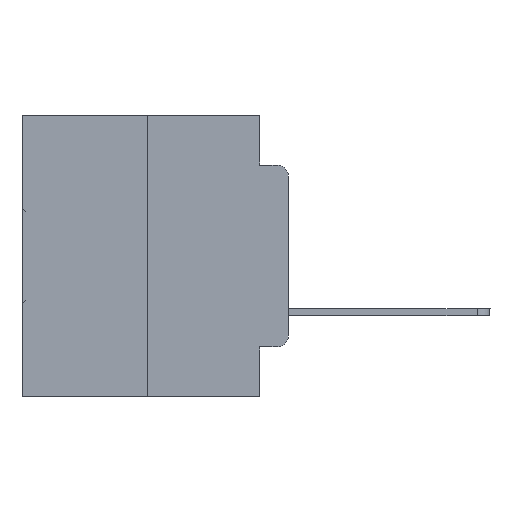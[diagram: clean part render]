
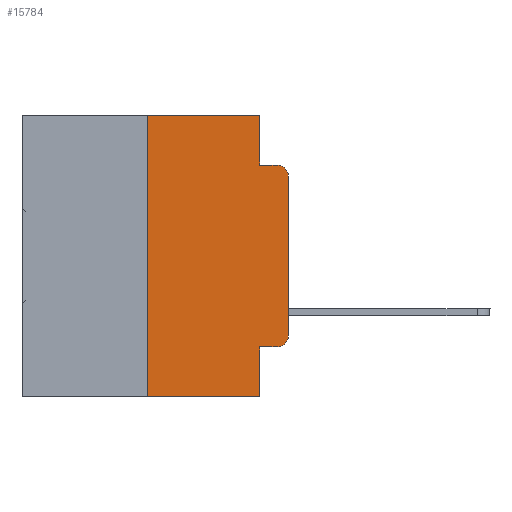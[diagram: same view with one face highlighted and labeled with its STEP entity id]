
A CAD part, left-side view. The second image highlights one B-rep face of the part: STEP entity #15784.
In plain terms, the highlighted planar face has unit normal (-1, 0, 0).
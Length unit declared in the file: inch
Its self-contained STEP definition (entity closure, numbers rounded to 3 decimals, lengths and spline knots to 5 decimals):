
#162 = VERTEX_POINT ( 'NONE', #5571 ) ;
#623 = LINE ( 'NONE', #5363, #6239 ) ;
#1288 = VERTEX_POINT ( 'NONE', #12887 ) ;
#1363 = AXIS2_PLACEMENT_3D ( 'NONE', #4456, #24964, #9524 ) ;
#1486 = VECTOR ( 'NONE', #15896, 39.37008 ) ;
#2655 = VERTEX_POINT ( 'NONE', #20567 ) ;
#3186 = CARTESIAN_POINT ( 'NONE',  ( 0., 0.051, 0. ) ) ;
#3588 = CIRCLE ( 'NONE', #24686, 0.02 ) ;
#3691 = VERTEX_POINT ( 'NONE', #13807 ) ;
#4365 = ORIENTED_EDGE ( 'NONE', *, *, #14681, .F. ) ;
#4456 = CARTESIAN_POINT ( 'NONE',  ( 0., 0.02, -0.3915 ) ) ;
#4658 = VECTOR ( 'NONE', #15212, 39.37008 ) ;
#4673 = CARTESIAN_POINT ( 'NONE',  ( 0., 0.051, -0.0885 ) ) ;
#4717 = VERTEX_POINT ( 'NONE', #15703 ) ;
#4820 = VECTOR ( 'NONE', #15538, 39.37008 ) ;
#4888 = EDGE_LOOP ( 'NONE', ( #22694, #17492, #4365, #20376, #17443, #29692, #32384, #18945, #14349, #13107 ) ) ;
#5183 = LINE ( 'NONE', #20302, #4820 ) ;
#5363 = CARTESIAN_POINT ( 'NONE',  ( 0., 0.051, -0.0885 ) ) ;
#5571 = CARTESIAN_POINT ( 'NONE',  ( 0., 0., -0.1085 ) ) ;
#6239 = VECTOR ( 'NONE', #21307, 39.37008 ) ;
#6391 = EDGE_CURVE ( 'NONE', #1288, #162, #12624, .T. ) ;
#7140 = DIRECTION ( 'NONE',  ( 1., 0., 0. ) ) ;
#7527 = DIRECTION ( 'NONE',  ( 0., 0., -1. ) ) ;
#7736 = CARTESIAN_POINT ( 'NONE',  ( 0., 0.473, 0. ) ) ;
#8259 = CARTESIAN_POINT ( 'NONE',  ( 0., 0.051, -0.4115 ) ) ;
#8658 = VECTOR ( 'NONE', #22796, 39.37008 ) ;
#9189 = VERTEX_POINT ( 'NONE', #19619 ) ;
#9524 = DIRECTION ( 'NONE',  ( 0., 0., -1. ) ) ;
#12209 = FACE_OUTER_BOUND ( 'NONE', #4888, .T. ) ;
#12624 = LINE ( 'NONE', #31084, #8658 ) ;
#12654 = CARTESIAN_POINT ( 'NONE',  ( 0., 0.051, 0. ) ) ;
#12887 = CARTESIAN_POINT ( 'NONE',  ( 0., 0., -0.3915 ) ) ;
#12994 = EDGE_CURVE ( 'NONE', #30410, #27808, #28955, .T. ) ;
#13107 = ORIENTED_EDGE ( 'NONE', *, *, #15301, .T. ) ;
#13537 = DIRECTION ( 'NONE',  ( 0., 0., -1. ) ) ;
#13544 = CARTESIAN_POINT ( 'NONE',  ( 0., 0.02, -0.4115 ) ) ;
#13807 = CARTESIAN_POINT ( 'NONE',  ( 0., 0.051, -0.4115 ) ) ;
#14231 = VERTEX_POINT ( 'NONE', #13544 ) ;
#14349 = ORIENTED_EDGE ( 'NONE', *, *, #17168, .T. ) ;
#14492 = DIRECTION ( 'NONE',  ( 0., -1., 0. ) ) ;
#14582 = CARTESIAN_POINT ( 'NONE',  ( 0., 0.051, 0. ) ) ;
#14681 = EDGE_CURVE ( 'NONE', #27808, #23661, #623, .T. ) ;
#15212 = DIRECTION ( 'NONE',  ( 0., 0., -1. ) ) ;
#15301 = EDGE_CURVE ( 'NONE', #14231, #1288, #31148, .T. ) ;
#15538 = DIRECTION ( 'NONE',  ( 0., 0., 1. ) ) ;
#15703 = CARTESIAN_POINT ( 'NONE',  ( 0., 0.25, 0. ) ) ;
#15784 = ADVANCED_FACE ( 'NONE', ( #12209 ), #22550, .F. ) ;
#15896 = DIRECTION ( 'NONE',  ( 0., -1., 0. ) ) ;
#17168 = EDGE_CURVE ( 'NONE', #3691, #14231, #26563, .T. ) ;
#17443 = ORIENTED_EDGE ( 'NONE', *, *, #21016, .F. ) ;
#17492 = ORIENTED_EDGE ( 'NONE', *, *, #29667, .T. ) ;
#17595 = CARTESIAN_POINT ( 'NONE',  ( 0., 0.02, -0.0885 ) ) ;
#18201 = VECTOR ( 'NONE', #13537, 39.37008 ) ;
#18945 = ORIENTED_EDGE ( 'NONE', *, *, #29339, .F. ) ;
#19619 = CARTESIAN_POINT ( 'NONE',  ( 0., 0.25, -0.5 ) ) ;
#19888 = EDGE_CURVE ( 'NONE', #9189, #4717, #5183, .T. ) ;
#19963 = LINE ( 'NONE', #7736, #32463 ) ;
#20297 = LINE ( 'NONE', #12654, #4658 ) ;
#20301 = DIRECTION ( 'NONE',  ( 0., -1., 0. ) ) ;
#20302 = CARTESIAN_POINT ( 'NONE',  ( 0., 0.25, 0. ) ) ;
#20376 = ORIENTED_EDGE ( 'NONE', *, *, #12994, .F. ) ;
#20567 = CARTESIAN_POINT ( 'NONE',  ( 0., 0.051, -0.5 ) ) ;
#21016 = EDGE_CURVE ( 'NONE', #4717, #30410, #19963, .T. ) ;
#21307 = DIRECTION ( 'NONE',  ( 0., -1., 0. ) ) ;
#21462 = VECTOR ( 'NONE', #14492, 39.37008 ) ;
#22550 = PLANE ( 'NONE',  #25220 ) ;
#22613 = CARTESIAN_POINT ( 'NONE',  ( 0., 0.473, -0.5 ) ) ;
#22694 = ORIENTED_EDGE ( 'NONE', *, *, #6391, .T. ) ;
#22796 = DIRECTION ( 'NONE',  ( 0., 0., 1. ) ) ;
#23661 = VERTEX_POINT ( 'NONE', #17595 ) ;
#24686 = AXIS2_PLACEMENT_3D ( 'NONE', #33271, #33442, #7527 ) ;
#24964 = DIRECTION ( 'NONE',  ( -1., 0., 0. ) ) ;
#25220 = AXIS2_PLACEMENT_3D ( 'NONE', #30355, #7140, #33051 ) ;
#26563 = LINE ( 'NONE', #8259, #1486 ) ;
#27702 = LINE ( 'NONE', #22613, #21462 ) ;
#27808 = VERTEX_POINT ( 'NONE', #4673 ) ;
#28955 = LINE ( 'NONE', #3186, #18201 ) ;
#29339 = EDGE_CURVE ( 'NONE', #3691, #2655, #20297, .T. ) ;
#29555 = EDGE_CURVE ( 'NONE', #9189, #2655, #27702, .T. ) ;
#29667 = EDGE_CURVE ( 'NONE', #162, #23661, #3588, .T. ) ;
#29692 = ORIENTED_EDGE ( 'NONE', *, *, #19888, .F. ) ;
#30355 = CARTESIAN_POINT ( 'NONE',  ( 0., 0.473, 0. ) ) ;
#30410 = VERTEX_POINT ( 'NONE', #14582 ) ;
#31084 = CARTESIAN_POINT ( 'NONE',  ( 0., 0., 0. ) ) ;
#31148 = CIRCLE ( 'NONE', #1363, 0.02 ) ;
#32384 = ORIENTED_EDGE ( 'NONE', *, *, #29555, .T. ) ;
#32463 = VECTOR ( 'NONE', #20301, 39.37008 ) ;
#33051 = DIRECTION ( 'NONE',  ( 0., 0., -1. ) ) ;
#33271 = CARTESIAN_POINT ( 'NONE',  ( 0., 0.02, -0.1085 ) ) ;
#33442 = DIRECTION ( 'NONE',  ( -1., 0., 0. ) ) ;
